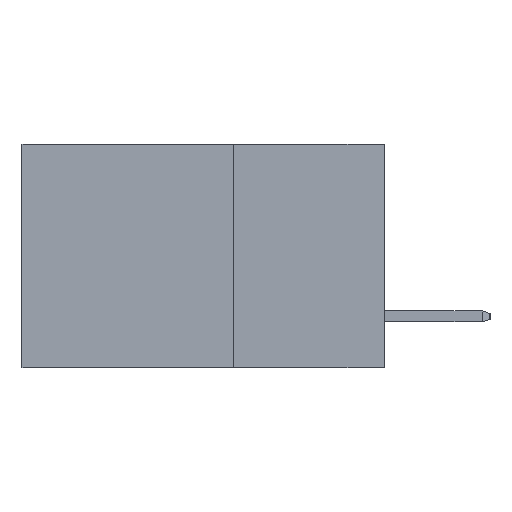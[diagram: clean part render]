
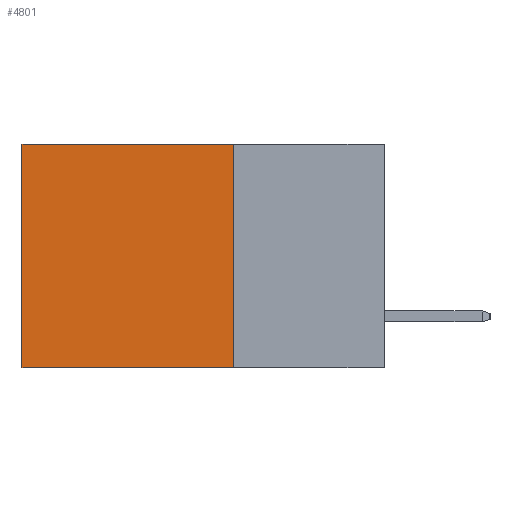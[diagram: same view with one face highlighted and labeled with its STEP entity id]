
A CAD part, left-side view. The second image highlights one B-rep face of the part: STEP entity #4801.
In plain terms, the highlighted planar face has unit normal (-1, 0, 0).
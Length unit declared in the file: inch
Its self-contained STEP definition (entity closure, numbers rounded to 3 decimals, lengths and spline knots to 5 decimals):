
#123 = VERTEX_POINT ( 'NONE', #6950 ) ;
#697 = VECTOR ( 'NONE', #4861, 39.37008 ) ;
#880 = DIRECTION ( 'NONE',  ( 0., 0., -1. ) ) ;
#918 = CARTESIAN_POINT ( 'NONE',  ( 0.2615, 0.6, 0. ) ) ;
#1196 = VECTOR ( 'NONE', #9148, 39.37008 ) ;
#1542 = VERTEX_POINT ( 'NONE', #918 ) ;
#1803 = CARTESIAN_POINT ( 'NONE',  ( 0.2615, 0.25, 0. ) ) ;
#2308 = ORIENTED_EDGE ( 'NONE', *, *, #4399, .T. ) ;
#2763 = AXIS2_PLACEMENT_3D ( 'NONE', #3010, #8206, #3744 ) ;
#3010 = CARTESIAN_POINT ( 'NONE',  ( 0.2615, 0.25, -0.37 ) ) ;
#3172 = LINE ( 'NONE', #4744, #1196 ) ;
#3744 = DIRECTION ( 'NONE',  ( 0., 0., -1. ) ) ;
#4096 = CARTESIAN_POINT ( 'NONE',  ( 0.2615, 0.6, -0.37 ) ) ;
#4104 = EDGE_LOOP ( 'NONE', ( #8109, #5611, #8328, #2308 ) ) ;
#4399 = EDGE_CURVE ( 'NONE', #4406, #1542, #3172, .T. ) ;
#4406 = VERTEX_POINT ( 'NONE', #1803 ) ;
#4744 = CARTESIAN_POINT ( 'NONE',  ( 0.2615, 0.25, 0. ) ) ;
#4801 = ADVANCED_FACE ( 'NONE', ( #4904 ), #6741, .F. ) ;
#4861 = DIRECTION ( 'NONE',  ( 0., 0., -1. ) ) ;
#4869 = VERTEX_POINT ( 'NONE', #6800 ) ;
#4904 = FACE_OUTER_BOUND ( 'NONE', #4104, .T. ) ;
#5363 = CARTESIAN_POINT ( 'NONE',  ( 0.2615, 0.25, -0.37 ) ) ;
#5611 = ORIENTED_EDGE ( 'NONE', *, *, #9295, .F. ) ;
#5815 = CARTESIAN_POINT ( 'NONE',  ( 0.2615, 0.25, -0.37 ) ) ;
#6667 = LINE ( 'NONE', #4096, #697 ) ;
#6741 = PLANE ( 'NONE',  #2763 ) ;
#6800 = CARTESIAN_POINT ( 'NONE',  ( 0.2615, 0.6, -0.37 ) ) ;
#6950 = CARTESIAN_POINT ( 'NONE',  ( 0.2615, 0.25, -0.37 ) ) ;
#7238 = LINE ( 'NONE', #5363, #9605 ) ;
#7460 = VECTOR ( 'NONE', #8774, 39.37008 ) ;
#7655 = EDGE_CURVE ( 'NONE', #1542, #4869, #6667, .T. ) ;
#8109 = ORIENTED_EDGE ( 'NONE', *, *, #7655, .T. ) ;
#8206 = DIRECTION ( 'NONE',  ( 1., 0., 0. ) ) ;
#8328 = ORIENTED_EDGE ( 'NONE', *, *, #8915, .F. ) ;
#8774 = DIRECTION ( 'NONE',  ( 0., 1., 0. ) ) ;
#8915 = EDGE_CURVE ( 'NONE', #4406, #123, #7238, .T. ) ;
#9148 = DIRECTION ( 'NONE',  ( 0., 1., 0. ) ) ;
#9295 = EDGE_CURVE ( 'NONE', #123, #4869, #9367, .T. ) ;
#9367 = LINE ( 'NONE', #5815, #7460 ) ;
#9605 = VECTOR ( 'NONE', #880, 39.37008 ) ;
